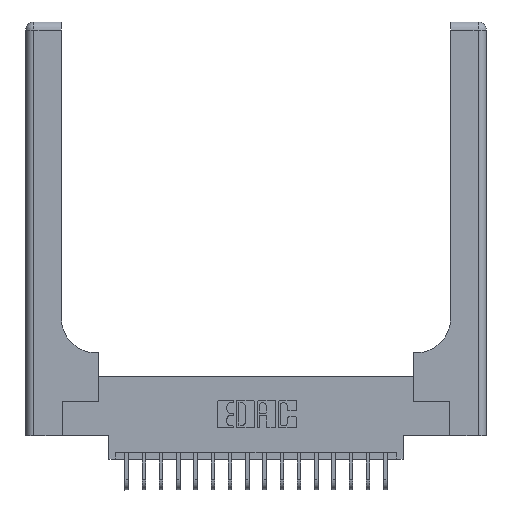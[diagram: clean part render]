
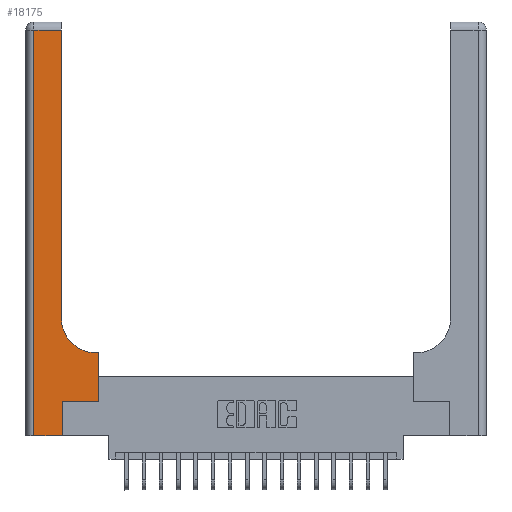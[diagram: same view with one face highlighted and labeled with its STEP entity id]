
A CAD part, top view. The second image highlights one B-rep face of the part: STEP entity #18175.
In plain terms, the highlighted planar face has unit normal (0, 0, 1).
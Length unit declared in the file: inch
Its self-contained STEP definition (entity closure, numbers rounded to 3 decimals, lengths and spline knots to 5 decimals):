
#11 = LINE ( 'NONE', #5592, #15301 ) ;
#64 = VECTOR ( 'NONE', #2342, 39.37008 ) ;
#183 = VERTEX_POINT ( 'NONE', #11330 ) ;
#238 = VERTEX_POINT ( 'NONE', #789 ) ;
#281 = VECTOR ( 'NONE', #13481, 39.37008 ) ;
#740 = VERTEX_POINT ( 'NONE', #2198 ) ;
#755 = EDGE_CURVE ( 'NONE', #8920, #15366, #11, .T. ) ;
#767 = DIRECTION ( 'NONE',  ( -1., 0., 0. ) ) ;
#789 = CARTESIAN_POINT ( 'NONE',  ( 0.06, 2.94, 0.37 ) ) ;
#839 = PLANE ( 'NONE',  #2474 ) ;
#974 = ORIENTED_EDGE ( 'NONE', *, *, #17639, .T. ) ;
#1014 = VECTOR ( 'NONE', #7018, 39.37008 ) ;
#1085 = CARTESIAN_POINT ( 'NONE',  ( 0.51, 0.85, 0.37 ) ) ;
#1359 = FACE_OUTER_BOUND ( 'NONE', #14766, .T. ) ;
#2198 = CARTESIAN_POINT ( 'NONE',  ( 0.528, 0.25, 0.37 ) ) ;
#2342 = DIRECTION ( 'NONE',  ( 0., 1., 0. ) ) ;
#2368 = VECTOR ( 'NONE', #20493, 39.37008 ) ;
#2474 = AXIS2_PLACEMENT_3D ( 'NONE', #9172, #4014, #767 ) ;
#2712 = DIRECTION ( 'NONE',  ( 0., 0., -1. ) ) ;
#2795 = LINE ( 'NONE', #19804, #10462 ) ;
#2908 = CARTESIAN_POINT ( 'NONE',  ( 0.265, 0.25, 0.37 ) ) ;
#3245 = CIRCLE ( 'NONE', #9403, 0.25 ) ;
#3403 = CARTESIAN_POINT ( 'NONE',  ( 0.265, 0.25, 0.37 ) ) ;
#3603 = DIRECTION ( 'NONE',  ( -1., 0., 0. ) ) ;
#3749 = CARTESIAN_POINT ( 'NONE',  ( 0.06, 3., 0.37 ) ) ;
#3904 = CARTESIAN_POINT ( 'NONE',  ( 0.51, 0.6, 0.37 ) ) ;
#4014 = DIRECTION ( 'NONE',  ( 0., 0., -1. ) ) ;
#4216 = CARTESIAN_POINT ( 'NONE',  ( 0., 2.94, 0.37 ) ) ;
#4332 = DIRECTION ( 'NONE',  ( 1., 0., 0. ) ) ;
#4367 = LINE ( 'NONE', #13465, #64 ) ;
#5592 = CARTESIAN_POINT ( 'NONE',  ( 0., 0., 0.37 ) ) ;
#5937 = ORIENTED_EDGE ( 'NONE', *, *, #20248, .T. ) ;
#6110 = LINE ( 'NONE', #4216, #7644 ) ;
#6251 = EDGE_CURVE ( 'NONE', #238, #8920, #11489, .T. ) ;
#6622 = CARTESIAN_POINT ( 'NONE',  ( 0.528, 0.6, 0.37 ) ) ;
#7018 = DIRECTION ( 'NONE',  ( 0., 1., 0. ) ) ;
#7119 = DIRECTION ( 'NONE',  ( 1., 0., 0. ) ) ;
#7411 = CARTESIAN_POINT ( 'NONE',  ( 0.265, 0., 0.37 ) ) ;
#7644 = VECTOR ( 'NONE', #14150, 39.37008 ) ;
#8143 = VECTOR ( 'NONE', #15453, 39.37008 ) ;
#8920 = VERTEX_POINT ( 'NONE', #10622 ) ;
#8927 = LINE ( 'NONE', #7411, #8143 ) ;
#9172 = CARTESIAN_POINT ( 'NONE',  ( 0., 3., 0.37 ) ) ;
#9403 = AXIS2_PLACEMENT_3D ( 'NONE', #1085, #2712, #4332 ) ;
#10462 = VECTOR ( 'NONE', #3603, 39.37008 ) ;
#10622 = CARTESIAN_POINT ( 'NONE',  ( 0.06, 0., 0.37 ) ) ;
#11330 = CARTESIAN_POINT ( 'NONE',  ( 0.26, 0.85, 0.37 ) ) ;
#11489 = LINE ( 'NONE', #3749, #281 ) ;
#11661 = ORIENTED_EDGE ( 'NONE', *, *, #12810, .T. ) ;
#12810 = EDGE_CURVE ( 'NONE', #17888, #14028, #2795, .T. ) ;
#13195 = EDGE_CURVE ( 'NONE', #15366, #15965, #8927, .T. ) ;
#13451 = CARTESIAN_POINT ( 'NONE',  ( 0.265, 0., 0.37 ) ) ;
#13465 = CARTESIAN_POINT ( 'NONE',  ( 0.528, 0.25, 0.37 ) ) ;
#13481 = DIRECTION ( 'NONE',  ( 0., -1., 0. ) ) ;
#13720 = EDGE_CURVE ( 'NONE', #13903, #238, #6110, .T. ) ;
#13903 = VERTEX_POINT ( 'NONE', #20037 ) ;
#14028 = VERTEX_POINT ( 'NONE', #3904 ) ;
#14150 = DIRECTION ( 'NONE',  ( -1., 0., 0. ) ) ;
#14250 = EDGE_CURVE ( 'NONE', #14028, #183, #3245, .T. ) ;
#14766 = EDGE_LOOP ( 'NONE', ( #5937, #18336, #15512, #20818, #15901, #974, #14911, #11661, #15014 ) ) ;
#14911 = ORIENTED_EDGE ( 'NONE', *, *, #17998, .T. ) ;
#15014 = ORIENTED_EDGE ( 'NONE', *, *, #14250, .T. ) ;
#15301 = VECTOR ( 'NONE', #7119, 39.37008 ) ;
#15338 = CARTESIAN_POINT ( 'NONE',  ( 0.26, 3., 0.37 ) ) ;
#15366 = VERTEX_POINT ( 'NONE', #13451 ) ;
#15453 = DIRECTION ( 'NONE',  ( 0., 1., 0. ) ) ;
#15512 = ORIENTED_EDGE ( 'NONE', *, *, #6251, .T. ) ;
#15901 = ORIENTED_EDGE ( 'NONE', *, *, #13195, .T. ) ;
#15965 = VERTEX_POINT ( 'NONE', #3403 ) ;
#16813 = LINE ( 'NONE', #15338, #1014 ) ;
#17639 = EDGE_CURVE ( 'NONE', #15965, #740, #20431, .T. ) ;
#17888 = VERTEX_POINT ( 'NONE', #6622 ) ;
#17998 = EDGE_CURVE ( 'NONE', #740, #17888, #4367, .T. ) ;
#18175 = ADVANCED_FACE ( 'NONE', ( #1359 ), #839, .F. ) ;
#18336 = ORIENTED_EDGE ( 'NONE', *, *, #13720, .T. ) ;
#19804 = CARTESIAN_POINT ( 'NONE',  ( 0.26, 0.6, 0.37 ) ) ;
#20037 = CARTESIAN_POINT ( 'NONE',  ( 0.26, 2.94, 0.37 ) ) ;
#20248 = EDGE_CURVE ( 'NONE', #183, #13903, #16813, .T. ) ;
#20431 = LINE ( 'NONE', #2908, #2368 ) ;
#20493 = DIRECTION ( 'NONE',  ( 1., 0., 0. ) ) ;
#20818 = ORIENTED_EDGE ( 'NONE', *, *, #755, .T. ) ;
